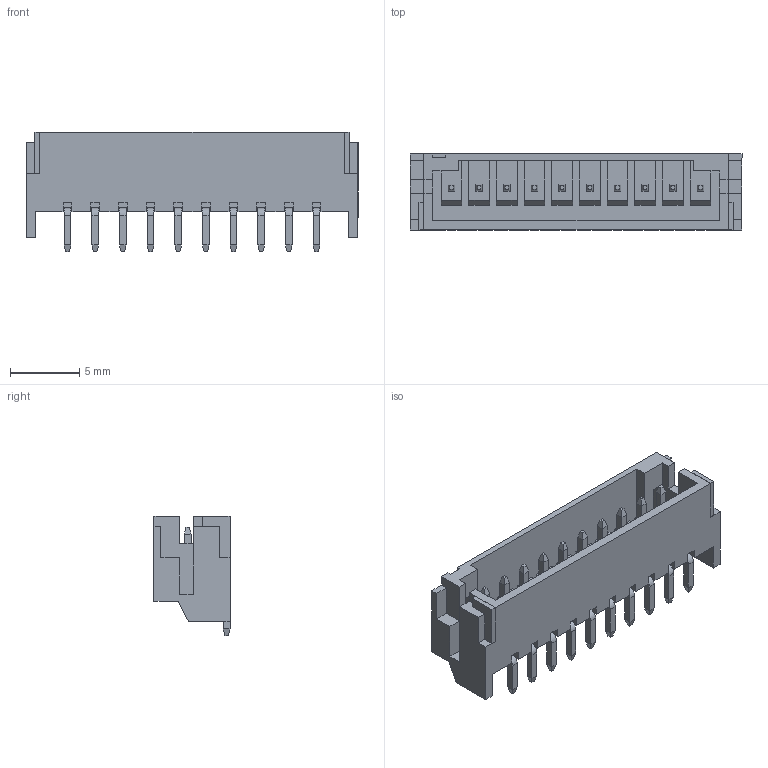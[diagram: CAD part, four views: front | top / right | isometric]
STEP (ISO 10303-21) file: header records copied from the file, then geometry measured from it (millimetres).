
FILE_DESCRIPTION (( 'STEP AP203' ), '1' );
FILE_NAME ('140-510-417-060.STEP', '2020-03-31T20:23:18', ( '' ), ( '' ), 'SwSTEP 2.0', 'SolidWorks 2016', '' );
FILE_SCHEMA (( 'CONFIG_CONTROL_DESIGN' ));
Length unit declared in the file: millimetre
Products named in the file (4): RA SMT Housing_510; RA SMT Contact; RA SMT Pad; 140-510-417-060
Assembly tree (13 placements, depth 2):
  140-510-417-060
    RA SMT Housing_510
    RA SMT Contact  x10
    RA SMT Pad  x2
Bounding box: 24 x 5.5 x 8.65 mm (x, y, z)
Volume: 327.7 mm3; surface area: 1235 mm2
Topology: 13 solids, 13 shells, 540 faces, 1312 edges, 794 vertices
Faces by surface type: plane 500, cylinder 40
Entity records: 9226 total; most frequent: CARTESIAN_POINT 1538, ORIENTED_EDGE 1520, DIRECTION 1328, EDGE_CURVE 760, LINE 752, VECTOR 752, VERTEX_POINT 498, AXIS2_PLACEMENT_3D 288
